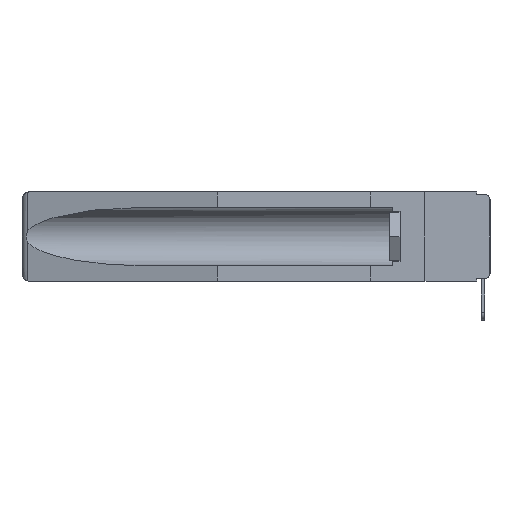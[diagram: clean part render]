
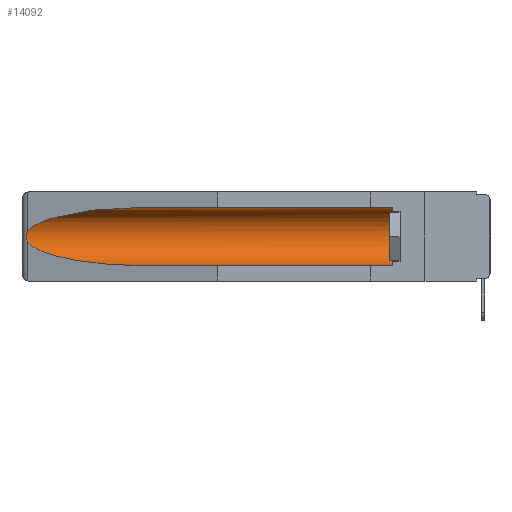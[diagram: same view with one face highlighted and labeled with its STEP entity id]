
A CAD part, left-side view. The second image highlights one B-rep face of the part: STEP entity #14092.
In plain terms, the highlighted cylindrical face has radius 2.857 mm (diameter 5.715 mm), a partial arc.
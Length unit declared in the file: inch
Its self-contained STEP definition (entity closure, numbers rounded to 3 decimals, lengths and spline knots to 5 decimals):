
#24 = EDGE_CURVE ( 'NONE', #9108, #15710, #3676, .T. ) ;
#858 = VECTOR ( 'NONE', #10159, 39.37008 ) ;
#1047 = CARTESIAN_POINT ( 'NONE',  ( 0.25451, 1.48313, -0.24835 ) ) ;
#1926 = CARTESIAN_POINT ( 'NONE',  ( 0.155, 1.07973, -0.059 ) ) ;
#1980 = CARTESIAN_POINT ( 'NONE',  ( 0.26537, 1.52718, -0.14972 ) ) ;
#2164 = EDGE_CURVE ( 'NONE', #18983, #4796, #19457, .T. ) ;
#2168 = AXIS2_PLACEMENT_3D ( 'NONE', #18510, #15831, #10899 ) ;
#3456 = CARTESIAN_POINT ( 'NONE',  ( 0.2673, 1.5327, -0.16383 ) ) ;
#3676 = B_SPLINE_CURVE_WITH_KNOTS ( 'NONE', 3,
 ( #12624, #9744, #6725, #3456, #6625, #8069, #12841, #12940, #4984, #15799 ),
 .UNSPECIFIED., .F., .F.,
 ( 4, 2, 2, 2, 4 ),
 ( 0., 0.00029, 0.00058, 0.00087, 0.00117 ),
 .UNSPECIFIED. ) ;
#4060 = LINE ( 'NONE', #6826, #858 ) ;
#4576 = DIRECTION ( 'NONE',  ( 0., -1., 0. ) ) ;
#4796 = VERTEX_POINT ( 'NONE', #5083 ) ;
#4804 = CYLINDRICAL_SURFACE ( 'NONE', #2168, 0.1125 ) ;
#4984 = CARTESIAN_POINT ( 'NONE',  ( 0.26597, 1.5296, -0.19026 ) ) ;
#5083 = CARTESIAN_POINT ( 'NONE',  ( 0.155, 0.126, -0.059 ) ) ;
#5742 = CARTESIAN_POINT ( 'NONE',  ( 0.155, 1.07973, -0.284 ) ) ;
#6625 = CARTESIAN_POINT ( 'NONE',  ( 0.2675, 1.53308, -0.16763 ) ) ;
#6725 = CARTESIAN_POINT ( 'NONE',  ( 0.26654, 1.53092, -0.15636 ) ) ;
#6826 = CARTESIAN_POINT ( 'NONE',  ( 0.155, -0.30754, -0.059 ) ) ;
#7741 = VECTOR ( 'NONE', #16635, 39.37008 ) ;
#7830 = EDGE_CURVE ( 'NONE', #14706, #9108, #19749, .T. ) ;
#8069 = CARTESIAN_POINT ( 'NONE',  ( 0.2675, 1.53308, -0.17534 ) ) ;
#8444 = CARTESIAN_POINT ( 'NONE',  ( 0.26537, 1.52718, -0.19328 ) ) ;
#8456 = CARTESIAN_POINT ( 'NONE',  ( 0.155, 0.126, -0.284 ) ) ;
#9108 = VERTEX_POINT ( 'NONE', #1980 ) ;
#9128 = FACE_OUTER_BOUND ( 'NONE', #18440, .T. ) ;
#9744 = CARTESIAN_POINT ( 'NONE',  ( 0.26597, 1.52961, -0.15275 ) ) ;
#9825 = CARTESIAN_POINT ( 'NONE',  ( 0.26537, 1.52718, -0.14972 ) ) ;
#9856 = ORIENTED_EDGE ( 'NONE', *, *, #2164, .T. ) ;
#10159 = DIRECTION ( 'NONE',  ( 0., 1., 0. ) ) ;
#10352 = LINE ( 'NONE', #13641, #7741 ) ;
#10584 = AXIS2_PLACEMENT_3D ( 'NONE', #12325, #4576, #15499 ) ;
#10597 = CARTESIAN_POINT ( 'NONE',  ( 0.21114, 1.30732, -0.284 ) ) ;
#10880 = CARTESIAN_POINT ( 'NONE',  ( 0.25451, 1.48313, -0.09465 ) ) ;
#10899 = DIRECTION ( 'NONE',  ( 0., 0., 1. ) ) ;
#11477 = ORIENTED_EDGE ( 'NONE', *, *, #13965, .T. ) ;
#11984 = ORIENTED_EDGE ( 'NONE', *, *, #7830, .T. ) ;
#12325 = CARTESIAN_POINT ( 'NONE',  ( 0.155, 0.126, -0.1715 ) ) ;
#12624 = CARTESIAN_POINT ( 'NONE',  ( 0.26537, 1.52718, -0.14972 ) ) ;
#12841 = CARTESIAN_POINT ( 'NONE',  ( 0.2673, 1.53269, -0.17917 ) ) ;
#12940 = CARTESIAN_POINT ( 'NONE',  ( 0.26655, 1.53094, -0.18657 ) ) ;
#13516 = EDGE_CURVE ( 'NONE', #4796, #14706, #4060, .T. ) ;
#13641 = CARTESIAN_POINT ( 'NONE',  ( 0.155, -0.30754, -0.284 ) ) ;
#13863 = CARTESIAN_POINT ( 'NONE',  ( 0.155, 1.07973, -0.284 ) ) ;
#13965 = EDGE_CURVE ( 'NONE', #15710, #20053, #18306, .T. ) ;
#14092 = ADVANCED_FACE ( 'NONE', ( #9128 ), #4804, .F. ) ;
#14706 = VERTEX_POINT ( 'NONE', #1926 ) ;
#14926 = CARTESIAN_POINT ( 'NONE',  ( 0.26537, 1.52718, -0.19328 ) ) ;
#14939 = EDGE_CURVE ( 'NONE', #18983, #20053, #10352, .T. ) ;
#15499 = DIRECTION ( 'NONE',  ( 0., 0., 1. ) ) ;
#15710 = VERTEX_POINT ( 'NONE', #8444 ) ;
#15799 = CARTESIAN_POINT ( 'NONE',  ( 0.26537, 1.52718, -0.19328 ) ) ;
#15831 = DIRECTION ( 'NONE',  ( 0., 1., 0. ) ) ;
#15990 = CARTESIAN_POINT ( 'NONE',  ( 0.21114, 1.30732, -0.059 ) ) ;
#16391 = ORIENTED_EDGE ( 'NONE', *, *, #13516, .T. ) ;
#16635 = DIRECTION ( 'NONE',  ( 0., 1., 0. ) ) ;
#18118 = ORIENTED_EDGE ( 'NONE', *, *, #14939, .F. ) ;
#18306 =( BOUNDED_CURVE ( )  B_SPLINE_CURVE ( 3, ( #14926, #1047, #10597, #5742 ),
 .UNSPECIFIED., .F., .F. ) 
 B_SPLINE_CURVE_WITH_KNOTS ( ( 4, 4 ),
 ( 0.1948, 1.5708 ),
 .UNSPECIFIED. ) 
 CURVE ( )  GEOMETRIC_REPRESENTATION_ITEM ( )  RATIONAL_B_SPLINE_CURVE ( ( 1., 0.848, 0.848, 1. ) ) 
 REPRESENTATION_ITEM ( '' )  );
#18440 = EDGE_LOOP ( 'NONE', ( #11984, #19951, #11477, #18118, #9856, #16391 ) ) ;
#18510 = CARTESIAN_POINT ( 'NONE',  ( 0.155, -0.30754, -0.1715 ) ) ;
#18689 = CARTESIAN_POINT ( 'NONE',  ( 0.155, 1.07973, -0.059 ) ) ;
#18983 = VERTEX_POINT ( 'NONE', #8456 ) ;
#19457 = CIRCLE ( 'NONE', #10584, 0.1125 ) ;
#19749 =( BOUNDED_CURVE ( )  B_SPLINE_CURVE ( 3, ( #18689, #15990, #10880, #9825 ),
 .UNSPECIFIED., .F., .F. ) 
 B_SPLINE_CURVE_WITH_KNOTS ( ( 4, 4 ),
 ( 4.71239, 6.08839 ),
 .UNSPECIFIED. ) 
 CURVE ( )  GEOMETRIC_REPRESENTATION_ITEM ( )  RATIONAL_B_SPLINE_CURVE ( ( 1., 0.848, 0.848, 1. ) ) 
 REPRESENTATION_ITEM ( '' )  );
#19951 = ORIENTED_EDGE ( 'NONE', *, *, #24, .T. ) ;
#20053 = VERTEX_POINT ( 'NONE', #13863 ) ;
